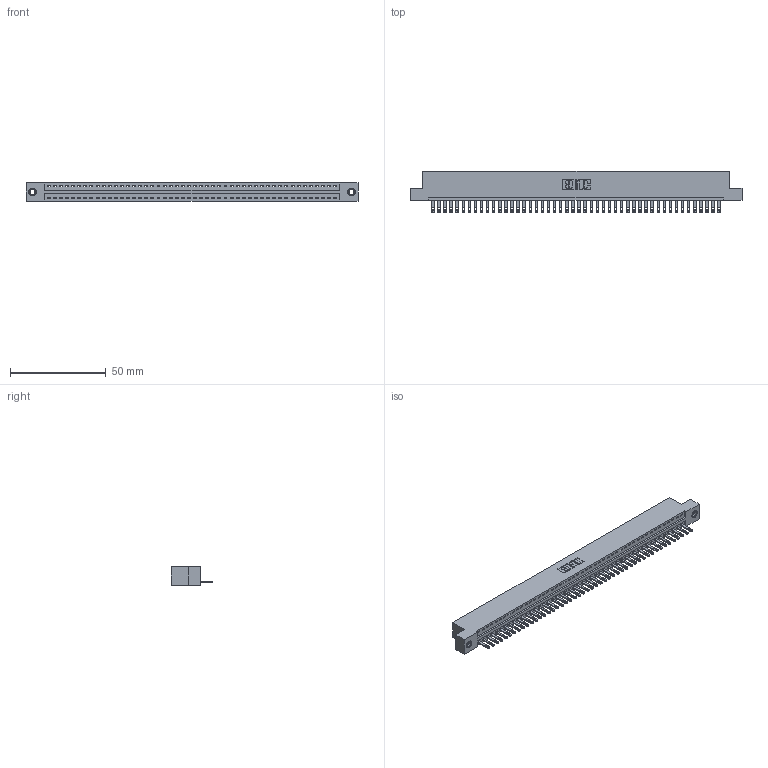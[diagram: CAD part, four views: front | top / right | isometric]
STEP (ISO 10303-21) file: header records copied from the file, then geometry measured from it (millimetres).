
FILE_DESCRIPTION (( 'STEP AP203' ), '1' );
FILE_NAME ('346-048-500-107.STEP', '2022-05-09T22:43:17', ( '' ), ( '' ), 'SwSTEP 2.0', 'SolidWorks 2020', '' );
FILE_SCHEMA (( 'CONFIG_CONTROL_DESIGN' ));
Length unit declared in the file: inch
Products named in the file (4): 346-048-500-107; 345-292-001_345-293-100; 346 Part_Flush Mounting Lugs - 0.156 Dia-TI; 345-250-001_345-250-005-103
Assembly tree (51 placements, depth 2):
  346-048-500-107
    346 Part_Flush Mounting Lugs - 0.156 Dia-TI
    345-292-001_345-293-100  x48
    345-250-001_345-250-005-103  x2
Bounding box: 172.97 x 21.84 x 9.4 mm (x, y, z)
Volume: 671 mm3; surface area: 18643.5 mm2
Topology: 50 solids, 51 shells, 2772 faces, 8529 edges, 5678 vertices
Faces by surface type: plane 1738, cylinder 1018, cone 12, torus 4
Entity records: 30098 total; most frequent: CARTESIAN_POINT 5139, ORIENTED_EDGE 5114, DIRECTION 4555, EDGE_CURVE 2557, LINE 2209, VECTOR 2209, VERTEX_POINT 1700, AXIS2_PLACEMENT_3D 1173
